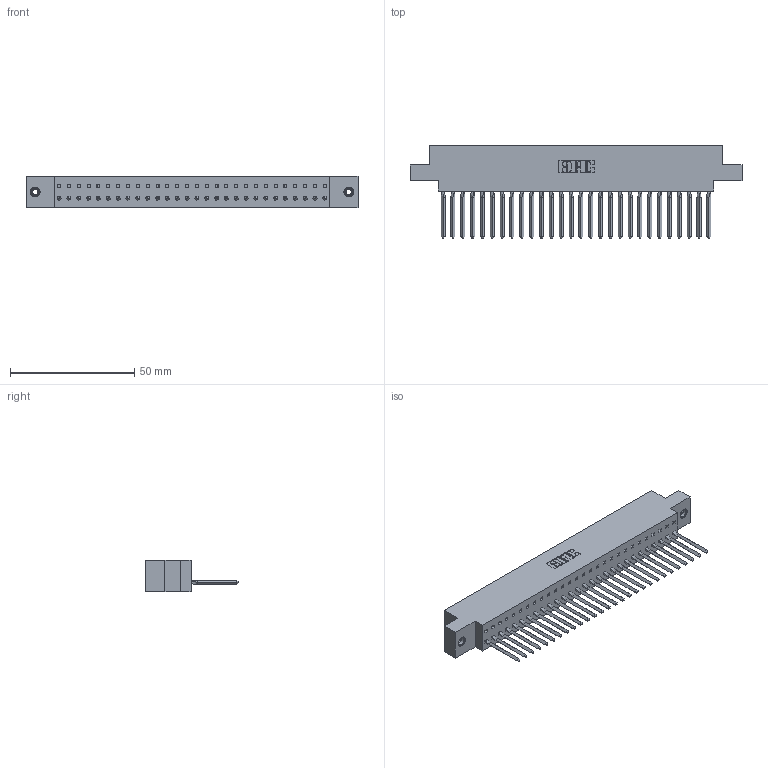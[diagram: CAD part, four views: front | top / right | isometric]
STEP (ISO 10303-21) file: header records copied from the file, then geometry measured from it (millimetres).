
FILE_DESCRIPTION (( 'STEP AP203' ), '1' );
FILE_NAME ('317-028-541-608.STEP', '2020-02-27T19:30:08', ( '' ), ( '' ), 'SwSTEP 2.0', 'SolidWorks 2016', '' );
FILE_SCHEMA (( 'CONFIG_CONTROL_DESIGN' ));
Length unit declared in the file: inch
Products named in the file (4): 345-250-001_345-250-003-102; 317-290-002_541; 317 Part_.156 Dia - TI; 317-028-541-608
Assembly tree (31 placements, depth 2):
  317-028-541-608
    317 Part_.156 Dia - TI
    317-290-002_541  x28
    345-250-001_345-250-003-102  x2
Bounding box: 133.65 x 37.34 x 12.7 mm (x, y, z)
Volume: 21237.3 mm3; surface area: 29564.5 mm2
Topology: 31 solids, 31 shells, 4418 faces, 12563 edges, 8162 vertices
Faces by surface type: plane 3562, cylinder 728, bspline 112, cone 12, torus 4
Entity records: 44265 total; most frequent: CARTESIAN_POINT 8472, ORIENTED_EDGE 7746, DIRECTION 6395, EDGE_CURVE 3873, LINE 3489, VECTOR 3489, VERTEX_POINT 2570, AXIS2_PLACEMENT_3D 1453
